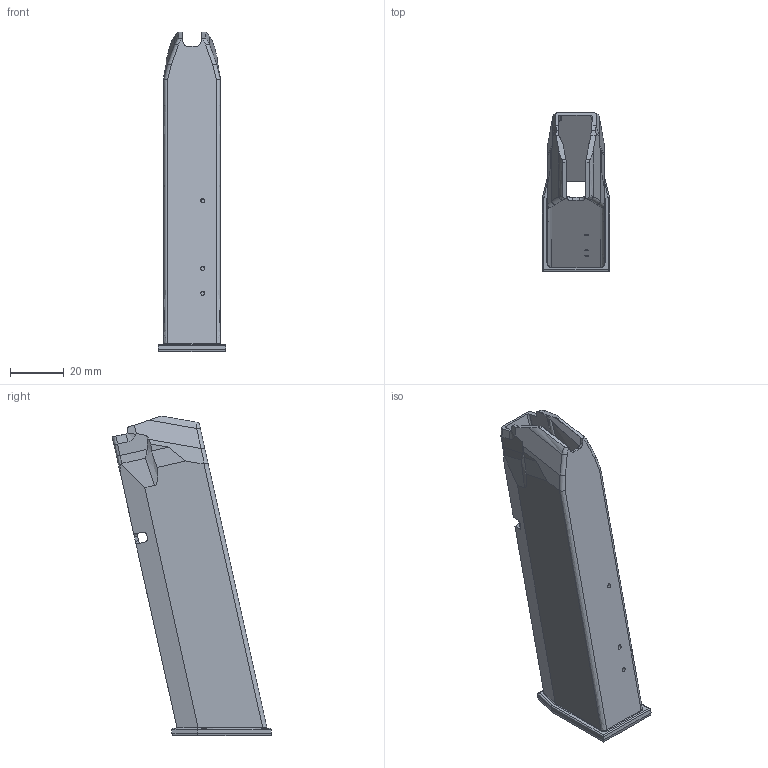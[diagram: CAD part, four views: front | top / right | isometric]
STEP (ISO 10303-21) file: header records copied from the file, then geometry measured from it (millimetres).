
FILE_DESCRIPTION(/* description */ (''),/* implementation_level */ '2;1');
FILE_NAME(/* name */ 'T-Mag17rd Ambi v1.1.step',/* time_stamp */ '2023-01-06T21:50:25-06:00',/* author */ (''),/* organization */ (''),/* preprocessor_version */ 'ST-DEVELOPER v19.2',/* originating_system */ 'Autodesk Translation Framework v11.17.0.187',/* authorisation */ '');
FILE_SCHEMA (('AUTOMOTIVE_DESIGN { 1 0 10303 214 3 1 1 }'));
Length unit declared in the file: millimetre
Products named in the file (1): T-Mag 17rd - v1
Bounding box: 24.97 x 59.31 x 118.93 mm (x, y, z)
Volume: 16939.8 mm3; surface area: 23855.5 mm2
Topology: 1 solids, 1 shells, 204 faces, 574 edges, 365 vertices
Faces by surface type: bspline 118, plane 85, cylinder 1
Entity records: 9658 total; most frequent: CARTESIAN_POINT 5000, ORIENTED_EDGE 1140, DIRECTION 709, EDGE_CURVE 570, VERTEX_POINT 365, LINE 279, VECTOR 279, AXIS2_PLACEMENT_3D 215
